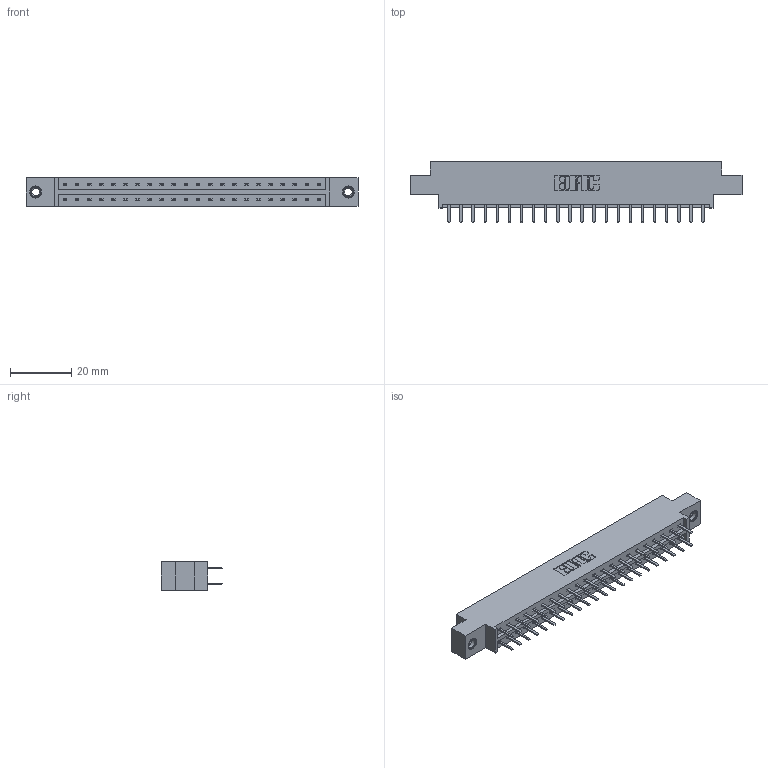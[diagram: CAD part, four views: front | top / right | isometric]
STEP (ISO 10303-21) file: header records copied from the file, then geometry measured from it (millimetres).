
FILE_DESCRIPTION (( 'STEP AP203' ), '1' );
FILE_NAME ('333-044-520-807.STEP', '2018-08-03T20:56:09', ( '' ), ( '' ), 'SwSTEP 2.0', 'SolidWorks 2016', '' );
FILE_SCHEMA (( 'CONFIG_CONTROL_DESIGN' ));
Length unit declared in the file: inch
Products named in the file (4): 345-292-001_345-293-120; 345-250-001_345-250-005-103; 333-044-520-807; 333 Part_Offset - .156 Dia - TI
Assembly tree (47 placements, depth 2):
  333-044-520-807
    333 Part_Offset - .156 Dia - TI
    345-292-001_345-293-120  x44
    345-250-001_345-250-005-103  x2
Bounding box: 108.71 x 20.02 x 9.4 mm (x, y, z)
Volume: 10651.2 mm3; surface area: 12581.2 mm2
Topology: 47 solids, 47 shells, 2642 faces, 7631 edges, 4962 vertices
Faces by surface type: plane 1778, cylinder 848, cone 12, torus 4
Entity records: 18172 total; most frequent: CARTESIAN_POINT 3033, ORIENTED_EDGE 2950, DIRECTION 2645, EDGE_CURVE 1475, LINE 1323, VECTOR 1323, VERTEX_POINT 976, AXIS2_PLACEMENT_3D 661
